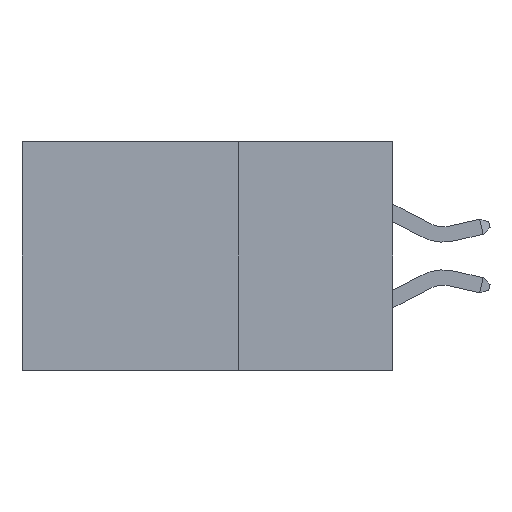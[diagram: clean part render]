
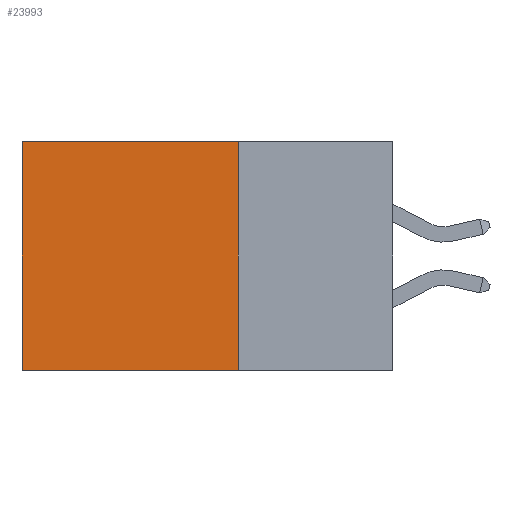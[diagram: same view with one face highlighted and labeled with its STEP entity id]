
A CAD part, left-side view. The second image highlights one B-rep face of the part: STEP entity #23993.
In plain terms, the highlighted planar face has unit normal (-1, 0, 0).
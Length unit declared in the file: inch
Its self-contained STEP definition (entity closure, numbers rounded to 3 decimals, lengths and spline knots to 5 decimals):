
#128 = CARTESIAN_POINT ( 'NONE',  ( 0.2875, 0.25, -0.37 ) ) ;
#534 = LINE ( 'NONE', #19573, #3045 ) ;
#1980 = VECTOR ( 'NONE', #29560, 39.37008 ) ;
#2347 = DIRECTION ( 'NONE',  ( 1., 0., 0. ) ) ;
#3045 = VECTOR ( 'NONE', #6174, 39.37008 ) ;
#3771 = ORIENTED_EDGE ( 'NONE', *, *, #31399, .F. ) ;
#4613 = CARTESIAN_POINT ( 'NONE',  ( 0.2875, 0.6, 0. ) ) ;
#5263 = VERTEX_POINT ( 'NONE', #24720 ) ;
#5904 = ORIENTED_EDGE ( 'NONE', *, *, #24151, .F. ) ;
#6174 = DIRECTION ( 'NONE',  ( 0., 0., -1. ) ) ;
#7402 = AXIS2_PLACEMENT_3D ( 'NONE', #12727, #2347, #21193 ) ;
#10781 = EDGE_LOOP ( 'NONE', ( #14198, #5904, #3771, #31255 ) ) ;
#10814 = LINE ( 'NONE', #35019, #1980 ) ;
#12610 = PLANE ( 'NONE',  #7402 ) ;
#12727 = CARTESIAN_POINT ( 'NONE',  ( 0.2875, 0.25, 0. ) ) ;
#13489 = VERTEX_POINT ( 'NONE', #19124 ) ;
#14198 = ORIENTED_EDGE ( 'NONE', *, *, #30696, .T. ) ;
#14275 = VECTOR ( 'NONE', #24528, 39.37008 ) ;
#19124 = CARTESIAN_POINT ( 'NONE',  ( 0.2875, 0.25, -0.37 ) ) ;
#19311 = EDGE_CURVE ( 'NONE', #32957, #20644, #10814, .T. ) ;
#19573 = CARTESIAN_POINT ( 'NONE',  ( 0.2875, 0.25, 0. ) ) ;
#19723 = DIRECTION ( 'NONE',  ( 0., 0., -1. ) ) ;
#19857 = FACE_OUTER_BOUND ( 'NONE', #10781, .T. ) ;
#20644 = VERTEX_POINT ( 'NONE', #4613 ) ;
#21193 = DIRECTION ( 'NONE',  ( 0., 0., -1. ) ) ;
#22219 = CARTESIAN_POINT ( 'NONE',  ( 0.2875, 0.6, 0. ) ) ;
#23993 = ADVANCED_FACE ( 'NONE', ( #19857 ), #12610, .F. ) ;
#24151 = EDGE_CURVE ( 'NONE', #13489, #5263, #27893, .T. ) ;
#24528 = DIRECTION ( 'NONE',  ( 0., 1., 0. ) ) ;
#24720 = CARTESIAN_POINT ( 'NONE',  ( 0.2875, 0.6, -0.37 ) ) ;
#26016 = LINE ( 'NONE', #22219, #32361 ) ;
#26729 = CARTESIAN_POINT ( 'NONE',  ( 0.2875, 0.25, 0. ) ) ;
#27893 = LINE ( 'NONE', #128, #14275 ) ;
#29560 = DIRECTION ( 'NONE',  ( 0., 1., 0. ) ) ;
#30696 = EDGE_CURVE ( 'NONE', #20644, #5263, #26016, .T. ) ;
#31255 = ORIENTED_EDGE ( 'NONE', *, *, #19311, .T. ) ;
#31399 = EDGE_CURVE ( 'NONE', #32957, #13489, #534, .T. ) ;
#32361 = VECTOR ( 'NONE', #19723, 39.37008 ) ;
#32957 = VERTEX_POINT ( 'NONE', #26729 ) ;
#35019 = CARTESIAN_POINT ( 'NONE',  ( 0.2875, 0.25, 0. ) ) ;
